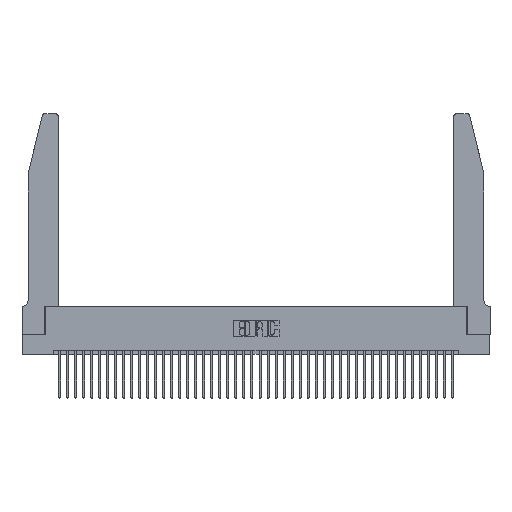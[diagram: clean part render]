
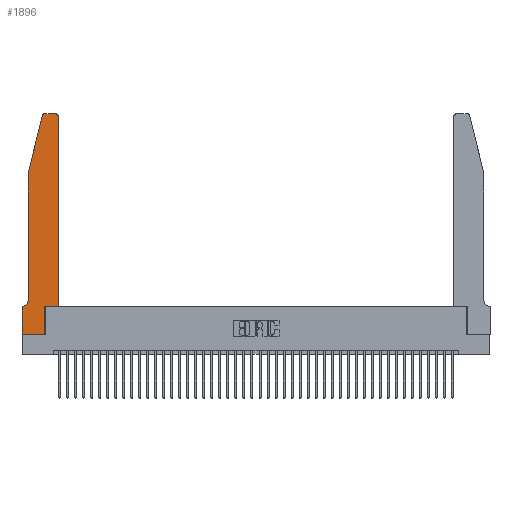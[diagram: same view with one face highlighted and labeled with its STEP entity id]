
A CAD part, top view. The second image highlights one B-rep face of the part: STEP entity #1896.
In plain terms, the highlighted planar face has unit normal (0, 0, 1).
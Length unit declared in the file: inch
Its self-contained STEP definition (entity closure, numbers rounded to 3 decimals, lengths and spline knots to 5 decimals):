
#197 = ORIENTED_EDGE ( 'NONE', *, *, #1341, .T. ) ;
#357 = ORIENTED_EDGE ( 'NONE', *, *, #9359, .T. ) ;
#1030 = DIRECTION ( 'NONE',  ( -0.239, -0.971, 0. ) ) ;
#1185 = DIRECTION ( 'NONE',  ( 0., 1., 0. ) ) ;
#1341 = EDGE_CURVE ( 'NONE', #42405, #3502, #34774, .T. ) ;
#1671 = ORIENTED_EDGE ( 'NONE', *, *, #2103, .T. ) ;
#1896 = ADVANCED_FACE ( 'NONE', ( #12947 ), #24862, .T. ) ;
#2103 = EDGE_CURVE ( 'NONE', #11280, #38585, #25646, .T. ) ;
#2427 = CARTESIAN_POINT ( 'NONE',  ( 0.284, 2.75, 0.37 ) ) ;
#2604 = DIRECTION ( 'NONE',  ( 1., 0., 0. ) ) ;
#3458 = VERTEX_POINT ( 'NONE', #8091 ) ;
#3502 = VERTEX_POINT ( 'NONE', #26225 ) ;
#4156 = ORIENTED_EDGE ( 'NONE', *, *, #39520, .T. ) ;
#4655 = EDGE_LOOP ( 'NONE', ( #6537, #4156, #9646, #39906, #38036, #357, #10302, #197, #21895, #26604, #1671, #13232 ) ) ;
#5706 = VECTOR ( 'NONE', #42717, 39.37008 ) ;
#6074 = CARTESIAN_POINT ( 'NONE',  ( 0.4205, 2.72, 0.37 ) ) ;
#6498 = VERTEX_POINT ( 'NONE', #35427 ) ;
#6537 = ORIENTED_EDGE ( 'NONE', *, *, #14303, .T. ) ;
#7656 = EDGE_CURVE ( 'NONE', #6498, #3458, #38695, .T. ) ;
#8091 = CARTESIAN_POINT ( 'NONE',  ( 0.0755, 2., 0.37 ) ) ;
#8242 = VECTOR ( 'NONE', #2604, 39.37008 ) ;
#8537 = DIRECTION ( 'NONE',  ( 0., -1., 0. ) ) ;
#9007 = DIRECTION ( 'NONE',  ( 0., 0., -1. ) ) ;
#9359 = EDGE_CURVE ( 'NONE', #10728, #40285, #11384, .T. ) ;
#9458 = CIRCLE ( 'NONE', #42370, 0.07 ) ;
#9510 = EDGE_CURVE ( 'NONE', #3502, #31425, #30502, .T. ) ;
#9541 = CARTESIAN_POINT ( 'NONE',  ( 0.0755, 0.42, 0.37 ) ) ;
#9646 = ORIENTED_EDGE ( 'NONE', *, *, #7656, .T. ) ;
#10302 = ORIENTED_EDGE ( 'NONE', *, *, #34274, .T. ) ;
#10728 = VERTEX_POINT ( 'NONE', #32829 ) ;
#10747 = CARTESIAN_POINT ( 'NONE',  ( 0.4505, 0.35, 0.37 ) ) ;
#11189 = VERTEX_POINT ( 'NONE', #32352 ) ;
#11280 = VERTEX_POINT ( 'NONE', #10747 ) ;
#11384 = LINE ( 'NONE', #31869, #36732 ) ;
#12006 = DIRECTION ( 'NONE',  ( 0., 0., 1. ) ) ;
#12751 = DIRECTION ( 'NONE',  ( -1., 0., 0. ) ) ;
#12947 = FACE_OUTER_BOUND ( 'NONE', #4655, .T. ) ;
#13037 = CARTESIAN_POINT ( 'NONE',  ( 0.2605, 2.75, 0.37 ) ) ;
#13092 = DIRECTION ( 'NONE',  ( 0., 1., 0. ) ) ;
#13232 = ORIENTED_EDGE ( 'NONE', *, *, #42695, .T. ) ;
#13786 = LINE ( 'NONE', #22424, #40192 ) ;
#14303 = EDGE_CURVE ( 'NONE', #11189, #35194, #27416, .T. ) ;
#16220 = AXIS2_PLACEMENT_3D ( 'NONE', #37747, #28062, #24410 ) ;
#18313 = LINE ( 'NONE', #31483, #30292 ) ;
#19495 = CARTESIAN_POINT ( 'NONE',  ( 0., 0., 0.37 ) ) ;
#20028 = VECTOR ( 'NONE', #1030, 39.37008 ) ;
#21393 = CARTESIAN_POINT ( 'NONE',  ( 0.284, 2.72, 0.37 ) ) ;
#21568 = CARTESIAN_POINT ( 'NONE',  ( 0.4505, 2.72, 0.37 ) ) ;
#21895 = ORIENTED_EDGE ( 'NONE', *, *, #9510, .T. ) ;
#22408 = CARTESIAN_POINT ( 'NONE',  ( 0.2865, 0.35, 0.37 ) ) ;
#22424 = CARTESIAN_POINT ( 'NONE',  ( 0.4505, 0.35, 0.37 ) ) ;
#22660 = CARTESIAN_POINT ( 'NONE',  ( 0., 0., 0.37 ) ) ;
#23351 = DIRECTION ( 'NONE',  ( 1., 0., 0. ) ) ;
#24410 = DIRECTION ( 'NONE',  ( 1., 0., 0. ) ) ;
#24862 = PLANE ( 'NONE',  #16220 ) ;
#24965 = CIRCLE ( 'NONE', #38455, 0.03 ) ;
#25005 = DIRECTION ( 'NONE',  ( -1., 0., 0. ) ) ;
#25646 = LINE ( 'NONE', #26650, #42256 ) ;
#25825 = DIRECTION ( 'NONE',  ( -1., 0., 0. ) ) ;
#26225 = CARTESIAN_POINT ( 'NONE',  ( 0.2865, 0., 0.37 ) ) ;
#26289 = EDGE_CURVE ( 'NONE', #31425, #11280, #13786, .T. ) ;
#26604 = ORIENTED_EDGE ( 'NONE', *, *, #26289, .T. ) ;
#26650 = CARTESIAN_POINT ( 'NONE',  ( 0.4505, 0.35, 0.37 ) ) ;
#27416 = LINE ( 'NONE', #13037, #32693 ) ;
#27848 = AXIS2_PLACEMENT_3D ( 'NONE', #21393, #12006, #34920 ) ;
#28062 = DIRECTION ( 'NONE',  ( 0., 0., 1. ) ) ;
#29754 = DIRECTION ( 'NONE',  ( 0., 0., 1. ) ) ;
#30292 = VECTOR ( 'NONE', #8537, 39.37008 ) ;
#30502 = LINE ( 'NONE', #34337, #32116 ) ;
#30678 = CARTESIAN_POINT ( 'NONE',  ( 0.0755, 2., 0.37 ) ) ;
#31425 = VERTEX_POINT ( 'NONE', #22408 ) ;
#31483 = CARTESIAN_POINT ( 'NONE',  ( 0.0755, 2., 0.37 ) ) ;
#31869 = CARTESIAN_POINT ( 'NONE',  ( 0.0755, 0.35, 0.37 ) ) ;
#32116 = VECTOR ( 'NONE', #1185, 39.37008 ) ;
#32149 = DIRECTION ( 'NONE',  ( 1., 0., 0. ) ) ;
#32352 = CARTESIAN_POINT ( 'NONE',  ( 0.4205, 2.75, 0.37 ) ) ;
#32599 = CIRCLE ( 'NONE', #27848, 0.03 ) ;
#32693 = VECTOR ( 'NONE', #12751, 39.37008 ) ;
#32829 = CARTESIAN_POINT ( 'NONE',  ( 0.0055, 0.35, 0.37 ) ) ;
#34274 = EDGE_CURVE ( 'NONE', #40285, #42405, #40482, .T. ) ;
#34337 = CARTESIAN_POINT ( 'NONE',  ( 0.2865, 0.35, 0.37 ) ) ;
#34774 = LINE ( 'NONE', #22660, #8242 ) ;
#34920 = DIRECTION ( 'NONE',  ( 1., 0., 0. ) ) ;
#35194 = VERTEX_POINT ( 'NONE', #2427 ) ;
#35427 = CARTESIAN_POINT ( 'NONE',  ( 0.25487, 2.72718, 0.37 ) ) ;
#36217 = EDGE_CURVE ( 'NONE', #3458, #38941, #18313, .T. ) ;
#36732 = VECTOR ( 'NONE', #25005, 39.37008 ) ;
#37747 = CARTESIAN_POINT ( 'NONE',  ( 0., 0.35, 0.37 ) ) ;
#38036 = ORIENTED_EDGE ( 'NONE', *, *, #42648, .T. ) ;
#38270 = CARTESIAN_POINT ( 'NONE',  ( 0., 0.35, 0.37 ) ) ;
#38455 = AXIS2_PLACEMENT_3D ( 'NONE', #6074, #29754, #23351 ) ;
#38585 = VERTEX_POINT ( 'NONE', #21568 ) ;
#38695 = LINE ( 'NONE', #30678, #20028 ) ;
#38941 = VERTEX_POINT ( 'NONE', #9541 ) ;
#39520 = EDGE_CURVE ( 'NONE', #35194, #6498, #32599, .T. ) ;
#39906 = ORIENTED_EDGE ( 'NONE', *, *, #36217, .T. ) ;
#40192 = VECTOR ( 'NONE', #32149, 39.37008 ) ;
#40285 = VERTEX_POINT ( 'NONE', #38270 ) ;
#40482 = LINE ( 'NONE', #19495, #5706 ) ;
#41360 = CARTESIAN_POINT ( 'NONE',  ( 0., 0., 0.37 ) ) ;
#42256 = VECTOR ( 'NONE', #13092, 39.37008 ) ;
#42370 = AXIS2_PLACEMENT_3D ( 'NONE', #42512, #9007, #25825 ) ;
#42405 = VERTEX_POINT ( 'NONE', #41360 ) ;
#42512 = CARTESIAN_POINT ( 'NONE',  ( 0.0055, 0.42, 0.37 ) ) ;
#42648 = EDGE_CURVE ( 'NONE', #38941, #10728, #9458, .T. ) ;
#42695 = EDGE_CURVE ( 'NONE', #38585, #11189, #24965, .T. ) ;
#42717 = DIRECTION ( 'NONE',  ( 0., -1., 0. ) ) ;
